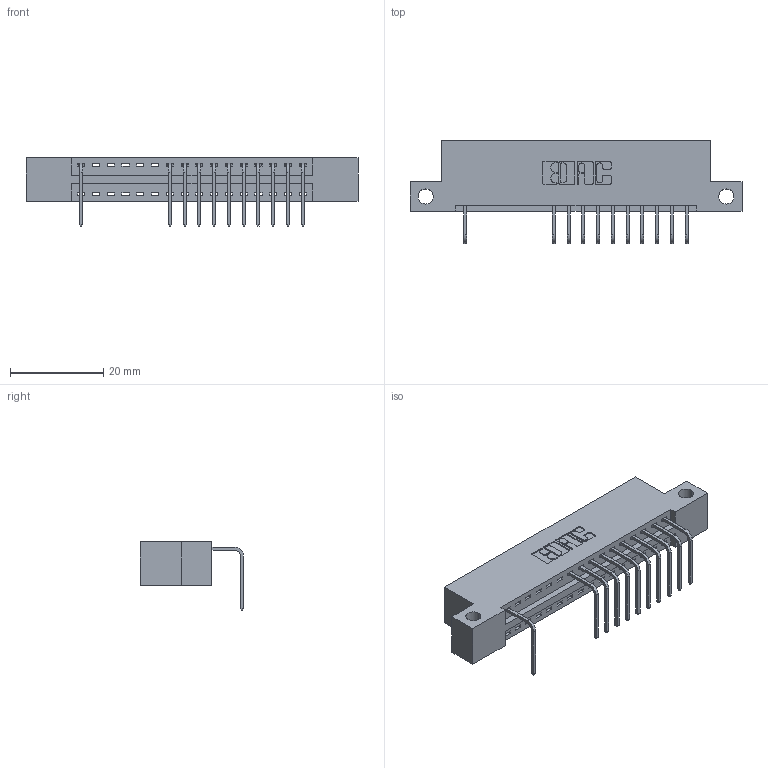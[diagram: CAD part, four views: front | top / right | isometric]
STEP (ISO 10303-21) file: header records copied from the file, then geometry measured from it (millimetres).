
FILE_DESCRIPTION (( 'STEP AP203' ), '1' );
FILE_NAME ('346-016-558-112.STEP', '2018-08-20T05:05:26', ( '' ), ( '' ), 'SwSTEP 2.0', 'SolidWorks 2016', '' );
FILE_SCHEMA (( 'CONFIG_CONTROL_DESIGN' ));
Length unit declared in the file: inch
Products named in the file (3): 346 Part_Flush Mounting Lugs - Side Mount; 345-292-001_558 Tail - 2; 346-016-558-112
Assembly tree (12 placements, depth 2):
  346-016-558-112
    346 Part_Flush Mounting Lugs - Side Mount
    345-292-001_558 Tail - 2  x11
Bounding box: 71.37 x 22.16 x 14.73 mm (x, y, z)
Volume: 6545.1 mm3; surface area: 7665.2 mm2
Topology: 12 solids, 12 shells, 842 faces, 2541 edges, 1678 vertices
Faces by surface type: plane 588, cylinder 254
Entity records: 13357 total; most frequent: CARTESIAN_POINT 2327, ORIENTED_EDGE 2282, DIRECTION 2079, EDGE_CURVE 1141, VECTOR 945, LINE 945, VERTEX_POINT 758, AXIS2_PLACEMENT_3D 567
